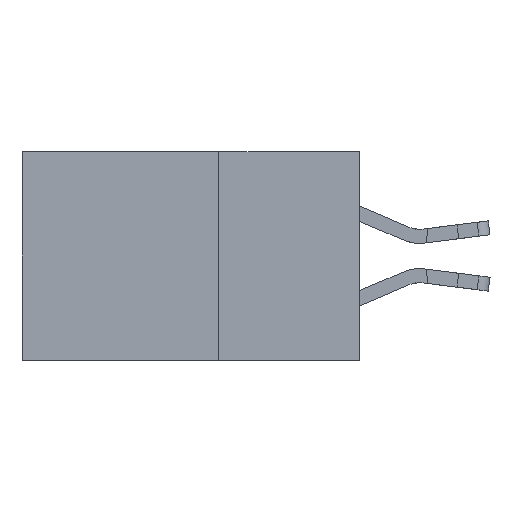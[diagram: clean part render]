
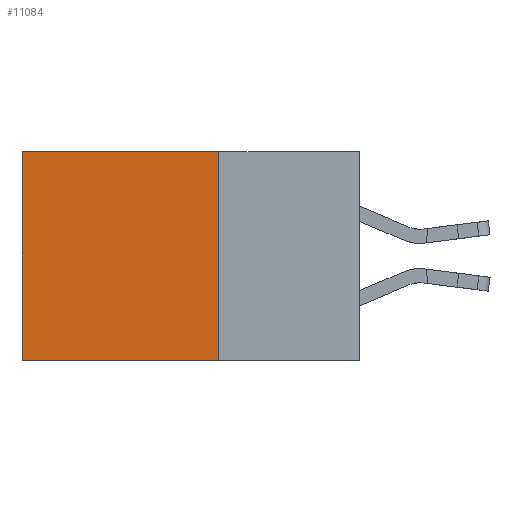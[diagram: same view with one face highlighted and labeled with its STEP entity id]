
A CAD part, left-side view. The second image highlights one B-rep face of the part: STEP entity #11084.
In plain terms, the highlighted planar face has unit normal (-1, 0, 0).
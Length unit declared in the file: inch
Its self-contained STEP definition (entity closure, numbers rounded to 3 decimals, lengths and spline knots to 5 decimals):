
#879 = CARTESIAN_POINT ( 'NONE',  ( 0.2875, 0.25, -0.37 ) ) ;
#1227 = CARTESIAN_POINT ( 'NONE',  ( 0.2875, 0.25, 0. ) ) ;
#2057 = EDGE_CURVE ( 'NONE', #10974, #27115, #19588, .T. ) ;
#2071 = ORIENTED_EDGE ( 'NONE', *, *, #8613, .T. ) ;
#3134 = DIRECTION ( 'NONE',  ( 0., 0., -1. ) ) ;
#4139 = ORIENTED_EDGE ( 'NONE', *, *, #19775, .F. ) ;
#4516 = VECTOR ( 'NONE', #3134, 39.37008 ) ;
#4982 = CARTESIAN_POINT ( 'NONE',  ( 0.2875, 0.6, 0. ) ) ;
#5336 = CARTESIAN_POINT ( 'NONE',  ( 0.2875, 0.25, 0. ) ) ;
#7562 = CARTESIAN_POINT ( 'NONE',  ( 0.2875, 0.6, 0. ) ) ;
#8103 = EDGE_LOOP ( 'NONE', ( #2071, #14482, #4139, #14676 ) ) ;
#8613 = EDGE_CURVE ( 'NONE', #12873, #27115, #14353, .T. ) ;
#9641 = DIRECTION ( 'NONE',  ( 0., 0., -1. ) ) ;
#9817 = PLANE ( 'NONE',  #11079 ) ;
#10388 = VECTOR ( 'NONE', #13525, 39.37008 ) ;
#10588 = VECTOR ( 'NONE', #22418, 39.37008 ) ;
#10974 = VERTEX_POINT ( 'NONE', #879 ) ;
#11079 = AXIS2_PLACEMENT_3D ( 'NONE', #1227, #22451, #9641 ) ;
#11084 = ADVANCED_FACE ( 'NONE', ( #12279 ), #9817, .F. ) ;
#12279 = FACE_OUTER_BOUND ( 'NONE', #8103, .T. ) ;
#12873 = VERTEX_POINT ( 'NONE', #7562 ) ;
#13525 = DIRECTION ( 'NONE',  ( 0., 1., 0. ) ) ;
#14353 = LINE ( 'NONE', #4982, #4516 ) ;
#14482 = ORIENTED_EDGE ( 'NONE', *, *, #2057, .F. ) ;
#14676 = ORIENTED_EDGE ( 'NONE', *, *, #18862, .T. ) ;
#15374 = LINE ( 'NONE', #5336, #10388 ) ;
#15604 = CARTESIAN_POINT ( 'NONE',  ( 0.2875, 0.25, 0. ) ) ;
#15700 = DIRECTION ( 'NONE',  ( 0., 0., -1. ) ) ;
#17347 = LINE ( 'NONE', #24298, #21007 ) ;
#18067 = CARTESIAN_POINT ( 'NONE',  ( 0.2875, 0.25, -0.37 ) ) ;
#18862 = EDGE_CURVE ( 'NONE', #23493, #12873, #15374, .T. ) ;
#19588 = LINE ( 'NONE', #18067, #10588 ) ;
#19775 = EDGE_CURVE ( 'NONE', #23493, #10974, #17347, .T. ) ;
#21007 = VECTOR ( 'NONE', #15700, 39.37008 ) ;
#22418 = DIRECTION ( 'NONE',  ( 0., 1., 0. ) ) ;
#22451 = DIRECTION ( 'NONE',  ( 1., 0., 0. ) ) ;
#23493 = VERTEX_POINT ( 'NONE', #15604 ) ;
#23603 = CARTESIAN_POINT ( 'NONE',  ( 0.2875, 0.6, -0.37 ) ) ;
#24298 = CARTESIAN_POINT ( 'NONE',  ( 0.2875, 0.25, 0. ) ) ;
#27115 = VERTEX_POINT ( 'NONE', #23603 ) ;
